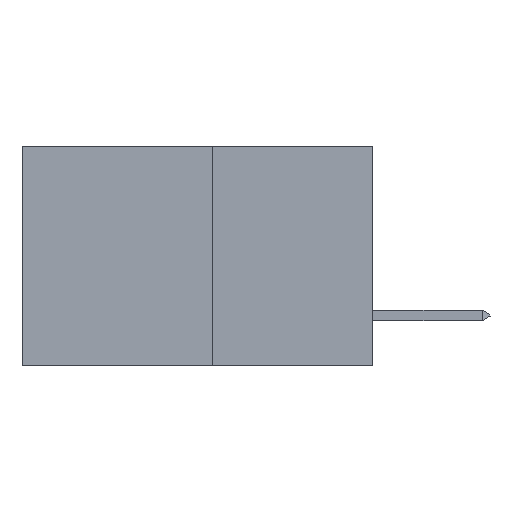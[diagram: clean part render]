
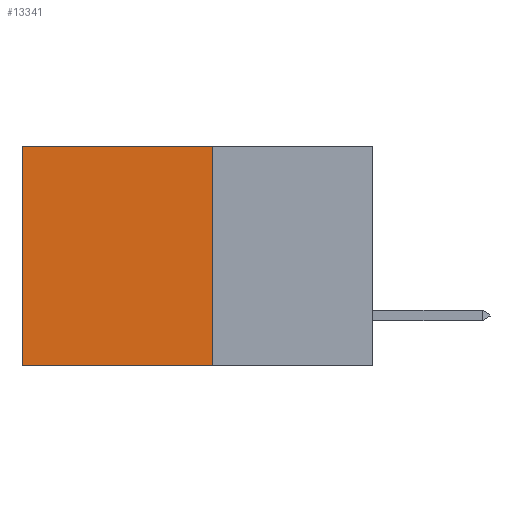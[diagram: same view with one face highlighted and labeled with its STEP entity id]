
A CAD part, left-side view. The second image highlights one B-rep face of the part: STEP entity #13341.
In plain terms, the highlighted planar face has unit normal (-1, 0, 0).
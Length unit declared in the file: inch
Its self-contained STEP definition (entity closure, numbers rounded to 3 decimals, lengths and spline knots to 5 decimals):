
#520 = EDGE_LOOP ( 'NONE', ( #7922, #7265, #13613, #7854 ) ) ;
#542 = CARTESIAN_POINT ( 'NONE',  ( 0.277, 0.27, -0.37 ) ) ;
#993 = CARTESIAN_POINT ( 'NONE',  ( 0.277, 0.59, 0. ) ) ;
#1068 = CARTESIAN_POINT ( 'NONE',  ( 0.277, 0.59, -0.37 ) ) ;
#2098 = CARTESIAN_POINT ( 'NONE',  ( 0.277, 0.59, -0.37 ) ) ;
#2841 = VERTEX_POINT ( 'NONE', #1068 ) ;
#3071 = VERTEX_POINT ( 'NONE', #13053 ) ;
#3342 = DIRECTION ( 'NONE',  ( 0., 0., -1. ) ) ;
#3360 = EDGE_CURVE ( 'NONE', #3071, #10219, #11888, .T. ) ;
#3861 = AXIS2_PLACEMENT_3D ( 'NONE', #542, #6853, #15502 ) ;
#4570 = CARTESIAN_POINT ( 'NONE',  ( 0.277, 0.27, -0.37 ) ) ;
#5032 = DIRECTION ( 'NONE',  ( 0., 1., 0. ) ) ;
#5398 = CARTESIAN_POINT ( 'NONE',  ( 0.277, 0.27, -0.37 ) ) ;
#5434 = VERTEX_POINT ( 'NONE', #5398 ) ;
#5567 = VECTOR ( 'NONE', #3342, 39.37008 ) ;
#5828 = DIRECTION ( 'NONE',  ( 0., 0., -1. ) ) ;
#6585 = EDGE_CURVE ( 'NONE', #5434, #2841, #13175, .T. ) ;
#6853 = DIRECTION ( 'NONE',  ( 1., 0., 0. ) ) ;
#7265 = ORIENTED_EDGE ( 'NONE', *, *, #6585, .F. ) ;
#7854 = ORIENTED_EDGE ( 'NONE', *, *, #3360, .T. ) ;
#7922 = ORIENTED_EDGE ( 'NONE', *, *, #7974, .T. ) ;
#7974 = EDGE_CURVE ( 'NONE', #10219, #2841, #15463, .T. ) ;
#8610 = VECTOR ( 'NONE', #9696, 39.37008 ) ;
#8920 = LINE ( 'NONE', #4570, #11433 ) ;
#9696 = DIRECTION ( 'NONE',  ( 0., 1., 0. ) ) ;
#9886 = VECTOR ( 'NONE', #5032, 39.37008 ) ;
#10219 = VERTEX_POINT ( 'NONE', #993 ) ;
#10506 = CARTESIAN_POINT ( 'NONE',  ( 0.277, 0.27, 0. ) ) ;
#11433 = VECTOR ( 'NONE', #5828, 39.37008 ) ;
#11888 = LINE ( 'NONE', #10506, #8610 ) ;
#12867 = EDGE_CURVE ( 'NONE', #3071, #5434, #8920, .T. ) ;
#12923 = CARTESIAN_POINT ( 'NONE',  ( 0.277, 0.27, -0.37 ) ) ;
#13027 = PLANE ( 'NONE',  #3861 ) ;
#13053 = CARTESIAN_POINT ( 'NONE',  ( 0.277, 0.27, 0. ) ) ;
#13175 = LINE ( 'NONE', #12923, #9886 ) ;
#13341 = ADVANCED_FACE ( 'NONE', ( #13529 ), #13027, .F. ) ;
#13529 = FACE_OUTER_BOUND ( 'NONE', #520, .T. ) ;
#13613 = ORIENTED_EDGE ( 'NONE', *, *, #12867, .F. ) ;
#15463 = LINE ( 'NONE', #2098, #5567 ) ;
#15502 = DIRECTION ( 'NONE',  ( 0., 0., -1. ) ) ;
